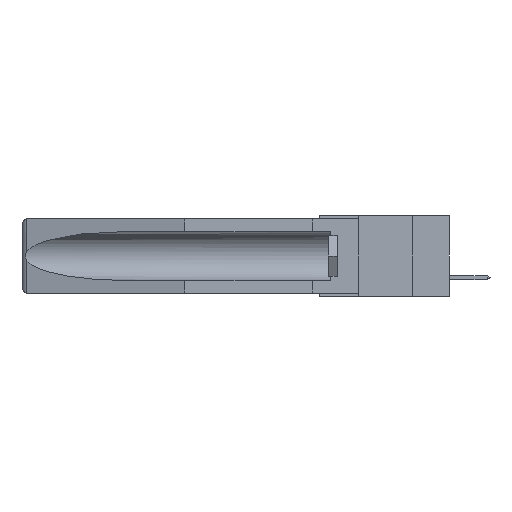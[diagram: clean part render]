
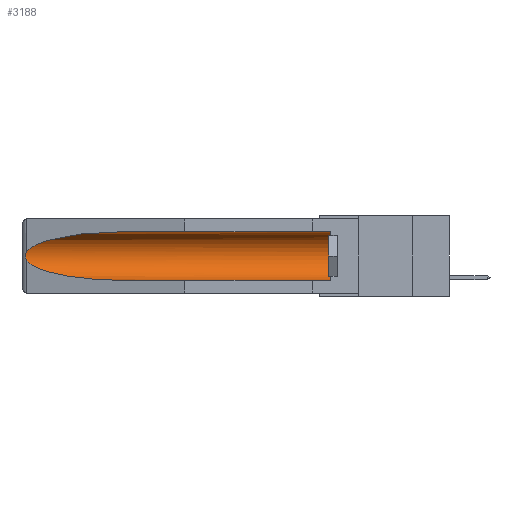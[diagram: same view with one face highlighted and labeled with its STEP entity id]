
A CAD part, left-side view. The second image highlights one B-rep face of the part: STEP entity #3188.
In plain terms, the highlighted cylindrical face has radius 2.857 mm (diameter 5.715 mm), a partial arc.
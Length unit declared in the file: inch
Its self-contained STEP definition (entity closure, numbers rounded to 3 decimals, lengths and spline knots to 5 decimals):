
#328 = CARTESIAN_POINT ( 'NONE',  ( 0.25451, 1.48313, -0.24835 ) ) ;
#531 = LINE ( 'NONE', #3725, #5986 ) ;
#762 = EDGE_CURVE ( 'NONE', #2282, #20238, #11722, .T. ) ;
#1323 = ORIENTED_EDGE ( 'NONE', *, *, #18528, .T. ) ;
#1609 = CARTESIAN_POINT ( 'NONE',  ( 0.155, -0.30754, -0.1715 ) ) ;
#1659 = B_SPLINE_CURVE_WITH_KNOTS ( 'NONE', 3,
 ( #11172, #1672, #15915, #17498, #6476, #19078, #9639, #11236, #1746, #12849 ),
 .UNSPECIFIED., .F., .F.,
 ( 4, 2, 2, 2, 4 ),
 ( 0., 0.00029, 0.00058, 0.00087, 0.00117 ),
 .UNSPECIFIED. ) ;
#1665 = VERTEX_POINT ( 'NONE', #13265 ) ;
#1672 = CARTESIAN_POINT ( 'NONE',  ( 0.26597, 1.52961, -0.15275 ) ) ;
#1746 = CARTESIAN_POINT ( 'NONE',  ( 0.26597, 1.5296, -0.19026 ) ) ;
#1949 = VERTEX_POINT ( 'NONE', #12301 ) ;
#2120 = ORIENTED_EDGE ( 'NONE', *, *, #762, .T. ) ;
#2282 = VERTEX_POINT ( 'NONE', #2283 ) ;
#2283 = CARTESIAN_POINT ( 'NONE',  ( 0.26537, 1.52718, -0.19328 ) ) ;
#2425 = EDGE_CURVE ( 'NONE', #6744, #2282, #1659, .T. ) ;
#2443 = CARTESIAN_POINT ( 'NONE',  ( 0.21114, 1.30732, -0.059 ) ) ;
#3188 = ADVANCED_FACE ( 'NONE', ( #8658 ), #18750, .F. ) ;
#3423 = CARTESIAN_POINT ( 'NONE',  ( 0.21114, 1.30732, -0.284 ) ) ;
#3725 = CARTESIAN_POINT ( 'NONE',  ( 0.155, -0.30754, -0.284 ) ) ;
#4542 = CARTESIAN_POINT ( 'NONE',  ( 0.155, 1.07973, -0.284 ) ) ;
#5331 = CARTESIAN_POINT ( 'NONE',  ( 0.155, 0.126, -0.1715 ) ) ;
#5986 = VECTOR ( 'NONE', #8656, 39.37008 ) ;
#6088 = CARTESIAN_POINT ( 'NONE',  ( 0.26537, 1.52718, -0.19328 ) ) ;
#6476 = CARTESIAN_POINT ( 'NONE',  ( 0.2675, 1.53308, -0.16763 ) ) ;
#6744 = VERTEX_POINT ( 'NONE', #15158 ) ;
#6897 = EDGE_CURVE ( 'NONE', #1949, #7676, #19096, .T. ) ;
#6930 = DIRECTION ( 'NONE',  ( 0., 0., 1. ) ) ;
#7322 = CARTESIAN_POINT ( 'NONE',  ( 0.155, 1.07973, -0.059 ) ) ;
#7676 = VERTEX_POINT ( 'NONE', #7322 ) ;
#8061 = DIRECTION ( 'NONE',  ( 0., 1., 0. ) ) ;
#8656 = DIRECTION ( 'NONE',  ( 0., 1., 0. ) ) ;
#8658 = FACE_OUTER_BOUND ( 'NONE', #10941, .T. ) ;
#8662 = EDGE_CURVE ( 'NONE', #1665, #20238, #531, .T. ) ;
#8750 = VECTOR ( 'NONE', #8061, 39.37008 ) ;
#9061 = EDGE_CURVE ( 'NONE', #1665, #1949, #18296, .T. ) ;
#9639 = CARTESIAN_POINT ( 'NONE',  ( 0.2673, 1.53269, -0.17917 ) ) ;
#10941 = EDGE_LOOP ( 'NONE', ( #1323, #18338, #2120, #12866, #15082, #19733 ) ) ;
#11172 = CARTESIAN_POINT ( 'NONE',  ( 0.26537, 1.52718, -0.14972 ) ) ;
#11236 = CARTESIAN_POINT ( 'NONE',  ( 0.26655, 1.53094, -0.18657 ) ) ;
#11722 =( BOUNDED_CURVE ( )  B_SPLINE_CURVE ( 3, ( #6088, #328, #3423, #4542 ),
 .UNSPECIFIED., .F., .T. ) 
 B_SPLINE_CURVE_WITH_KNOTS ( ( 4, 4 ),
 ( 0.1948, 1.5708 ),
 .UNSPECIFIED. ) 
 CURVE ( )  GEOMETRIC_REPRESENTATION_ITEM ( )  RATIONAL_B_SPLINE_CURVE ( ( 1., 0.848, 0.848, 1. ) ) 
 REPRESENTATION_ITEM ( '' )  );
#12301 = CARTESIAN_POINT ( 'NONE',  ( 0.155, 0.126, -0.059 ) ) ;
#12716 = DIRECTION ( 'NONE',  ( 0., 0., 1. ) ) ;
#12849 = CARTESIAN_POINT ( 'NONE',  ( 0.26537, 1.52718, -0.19328 ) ) ;
#12866 = ORIENTED_EDGE ( 'NONE', *, *, #8662, .F. ) ;
#13265 = CARTESIAN_POINT ( 'NONE',  ( 0.155, 0.126, -0.284 ) ) ;
#13444 = CARTESIAN_POINT ( 'NONE',  ( 0.155, 1.07973, -0.284 ) ) ;
#14863 = DIRECTION ( 'NONE',  ( 0., -1., 0. ) ) ;
#15082 = ORIENTED_EDGE ( 'NONE', *, *, #9061, .T. ) ;
#15158 = CARTESIAN_POINT ( 'NONE',  ( 0.26537, 1.52718, -0.14972 ) ) ;
#15575 = DIRECTION ( 'NONE',  ( 0., 1., 0. ) ) ;
#15915 = CARTESIAN_POINT ( 'NONE',  ( 0.26654, 1.53092, -0.15636 ) ) ;
#16050 = CARTESIAN_POINT ( 'NONE',  ( 0.155, -0.30754, -0.059 ) ) ;
#16463 = CARTESIAN_POINT ( 'NONE',  ( 0.155, 1.07973, -0.059 ) ) ;
#16598 = CARTESIAN_POINT ( 'NONE',  ( 0.26537, 1.52718, -0.14972 ) ) ;
#16980 =( BOUNDED_CURVE ( )  B_SPLINE_CURVE ( 3, ( #16463, #2443, #19609, #16598 ),
 .UNSPECIFIED., .F., .F. ) 
 B_SPLINE_CURVE_WITH_KNOTS ( ( 4, 4 ),
 ( 4.71239, 6.08839 ),
 .UNSPECIFIED. ) 
 CURVE ( )  GEOMETRIC_REPRESENTATION_ITEM ( )  RATIONAL_B_SPLINE_CURVE ( ( 1., 0.848, 0.848, 1. ) ) 
 REPRESENTATION_ITEM ( '' )  );
#17498 = CARTESIAN_POINT ( 'NONE',  ( 0.2673, 1.5327, -0.16383 ) ) ;
#17549 = AXIS2_PLACEMENT_3D ( 'NONE', #1609, #15575, #12716 ) ;
#18296 = CIRCLE ( 'NONE', #19596, 0.1125 ) ;
#18338 = ORIENTED_EDGE ( 'NONE', *, *, #2425, .T. ) ;
#18528 = EDGE_CURVE ( 'NONE', #7676, #6744, #16980, .T. ) ;
#18750 = CYLINDRICAL_SURFACE ( 'NONE', #17549, 0.1125 ) ;
#19078 = CARTESIAN_POINT ( 'NONE',  ( 0.2675, 1.53308, -0.17534 ) ) ;
#19096 = LINE ( 'NONE', #16050, #8750 ) ;
#19596 = AXIS2_PLACEMENT_3D ( 'NONE', #5331, #14863, #6930 ) ;
#19609 = CARTESIAN_POINT ( 'NONE',  ( 0.25451, 1.48313, -0.09465 ) ) ;
#19733 = ORIENTED_EDGE ( 'NONE', *, *, #6897, .T. ) ;
#20238 = VERTEX_POINT ( 'NONE', #13444 ) ;
